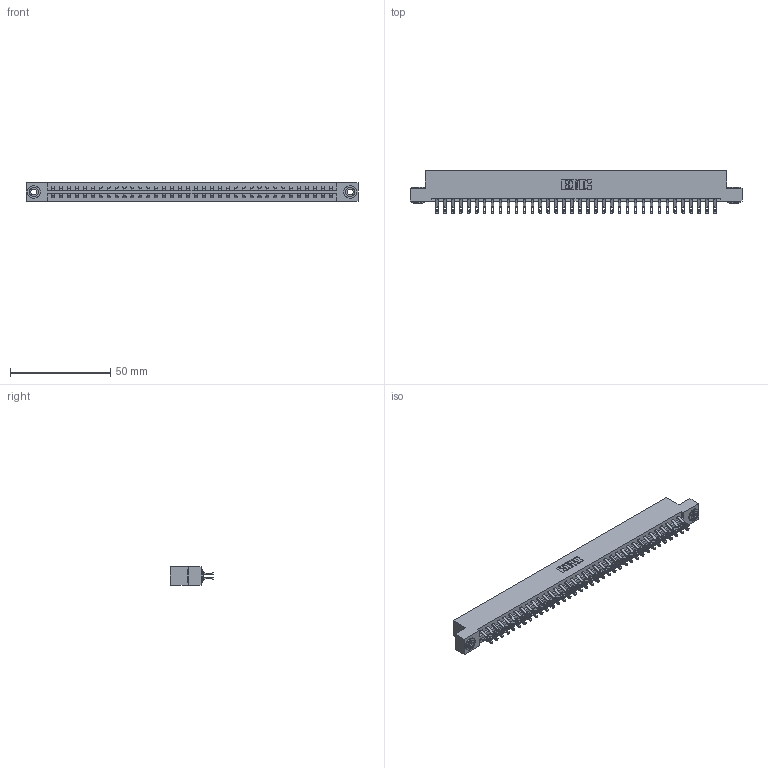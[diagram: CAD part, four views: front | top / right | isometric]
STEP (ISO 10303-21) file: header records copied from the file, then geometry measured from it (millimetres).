
FILE_DESCRIPTION (( 'STEP AP203' ), '1' );
FILE_NAME ('337-072-555-203.STEP', '2018-08-11T15:18:28', ( '' ), ( '' ), 'SwSTEP 2.0', 'SolidWorks 2016', '' );
FILE_SCHEMA (( 'CONFIG_CONTROL_DESIGN' ));
Length unit declared in the file: inch
Products named in the file (4): 337 Part_Flush Mounting Lugs - 0.156 Dia-TH; 345-292-001_555 Tail; 345-250-002_345-250-002-102; 337-072-555-203
Assembly tree (75 placements, depth 2):
  337-072-555-203
    337 Part_Flush Mounting Lugs - 0.156 Dia-TH
    345-292-001_555 Tail  x72
    345-250-002_345-250-002-102  x2
Bounding box: 165.66 x 21.47 x 9.4 mm (x, y, z)
Volume: 17606.8 mm3; surface area: 20857.7 mm2
Topology: 75 solids, 75 shells, 4472 faces, 13995 edges, 9326 vertices
Faces by surface type: plane 2672, cylinder 1792, cone 8
Entity records: 29664 total; most frequent: CARTESIAN_POINT 5011, ORIENTED_EDGE 4910, DIRECTION 4277, EDGE_CURVE 2455, VECTOR 2283, LINE 2283, VERTEX_POINT 1634, AXIS2_PLACEMENT_3D 997
